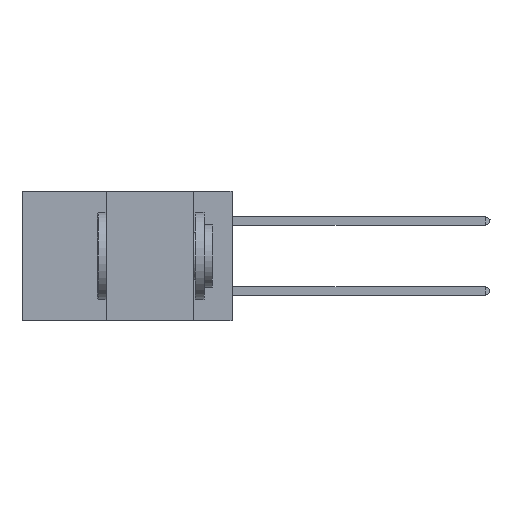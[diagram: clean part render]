
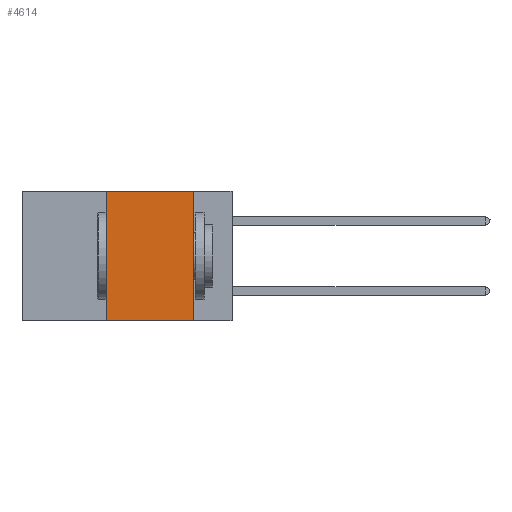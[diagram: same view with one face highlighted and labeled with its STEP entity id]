
A CAD part, left-side view. The second image highlights one B-rep face of the part: STEP entity #4614.
In plain terms, the highlighted planar face has unit normal (-1, 0, 0).
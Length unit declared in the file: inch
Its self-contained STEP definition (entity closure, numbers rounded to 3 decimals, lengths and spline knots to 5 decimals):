
#930 = ORIENTED_EDGE ( 'NONE', *, *, #28788, .F. ) ;
#2730 = LINE ( 'NONE', #23301, #18300 ) ;
#4614 = ADVANCED_FACE ( 'NONE', ( #29325 ), #14622, .F. ) ;
#5719 = CARTESIAN_POINT ( 'NONE',  ( 0., 0.36, 0. ) ) ;
#6764 = DIRECTION ( 'NONE',  ( 0., -1., 0. ) ) ;
#7236 = AXIS2_PLACEMENT_3D ( 'NONE', #21853, #32155, #29370 ) ;
#9660 = VERTEX_POINT ( 'NONE', #11639 ) ;
#11639 = CARTESIAN_POINT ( 'NONE',  ( 0., 0.36, -0.37 ) ) ;
#13347 = DIRECTION ( 'NONE',  ( 0., 0., -1. ) ) ;
#14622 = PLANE ( 'NONE',  #7236 ) ;
#14862 = VERTEX_POINT ( 'NONE', #5719 ) ;
#15701 = EDGE_CURVE ( 'NONE', #14862, #20140, #31210, .T. ) ;
#16671 = CARTESIAN_POINT ( 'NONE',  ( 0., 0.6, 0. ) ) ;
#18300 = VECTOR ( 'NONE', #13347, 39.37008 ) ;
#18553 = CARTESIAN_POINT ( 'NONE',  ( 0., 0.11, -0.37 ) ) ;
#19206 = VERTEX_POINT ( 'NONE', #18553 ) ;
#19594 = DIRECTION ( 'NONE',  ( 0., 0., 1. ) ) ;
#19651 = DIRECTION ( 'NONE',  ( 0., -1., 0. ) ) ;
#19899 = ORIENTED_EDGE ( 'NONE', *, *, #32014, .T. ) ;
#20140 = VERTEX_POINT ( 'NONE', #21048 ) ;
#21048 = CARTESIAN_POINT ( 'NONE',  ( 0., 0.11, 0. ) ) ;
#21425 = EDGE_LOOP ( 'NONE', ( #930, #24180, #21871, #19899 ) ) ;
#21853 = CARTESIAN_POINT ( 'NONE',  ( 0., 0.6, 0. ) ) ;
#21871 = ORIENTED_EDGE ( 'NONE', *, *, #22423, .F. ) ;
#22408 = VECTOR ( 'NONE', #19651, 39.37008 ) ;
#22423 = EDGE_CURVE ( 'NONE', #9660, #14862, #22784, .T. ) ;
#22784 = LINE ( 'NONE', #24089, #24739 ) ;
#22787 = LINE ( 'NONE', #27412, #22408 ) ;
#23301 = CARTESIAN_POINT ( 'NONE',  ( 0., 0.11, 0. ) ) ;
#24089 = CARTESIAN_POINT ( 'NONE',  ( 0., 0.36, 0. ) ) ;
#24180 = ORIENTED_EDGE ( 'NONE', *, *, #15701, .F. ) ;
#24609 = VECTOR ( 'NONE', #6764, 39.37008 ) ;
#24739 = VECTOR ( 'NONE', #19594, 39.37008 ) ;
#27412 = CARTESIAN_POINT ( 'NONE',  ( 0., 0.6, -0.37 ) ) ;
#28788 = EDGE_CURVE ( 'NONE', #20140, #19206, #2730, .T. ) ;
#29325 = FACE_OUTER_BOUND ( 'NONE', #21425, .T. ) ;
#29370 = DIRECTION ( 'NONE',  ( 0., 0., -1. ) ) ;
#31210 = LINE ( 'NONE', #16671, #24609 ) ;
#32014 = EDGE_CURVE ( 'NONE', #9660, #19206, #22787, .T. ) ;
#32155 = DIRECTION ( 'NONE',  ( 1., 0., 0. ) ) ;
